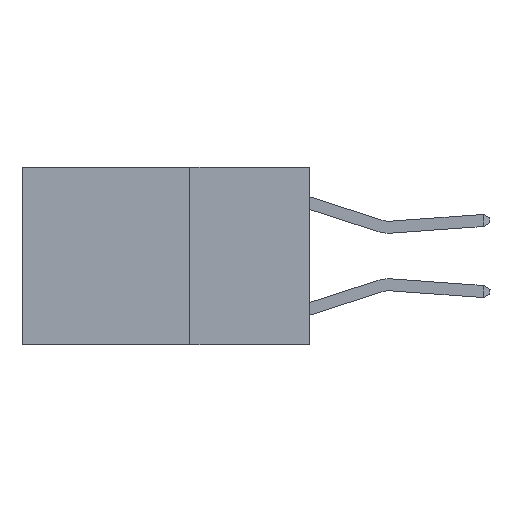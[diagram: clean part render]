
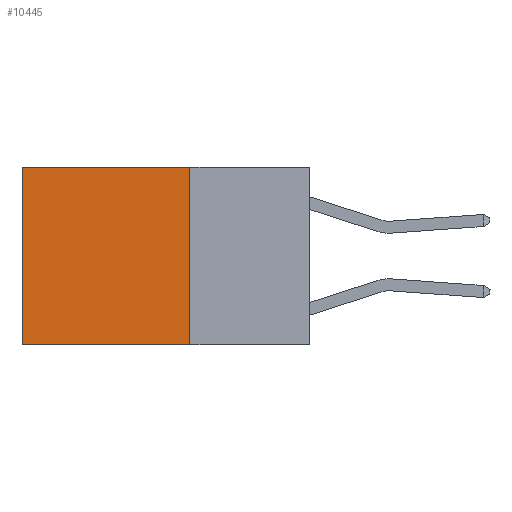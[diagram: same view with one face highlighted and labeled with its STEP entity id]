
A CAD part, left-side view. The second image highlights one B-rep face of the part: STEP entity #10445.
In plain terms, the highlighted planar face has unit normal (-1, 0, 0).
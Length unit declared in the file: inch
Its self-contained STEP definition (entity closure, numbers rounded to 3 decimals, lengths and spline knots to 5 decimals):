
#79 = CARTESIAN_POINT ( 'NONE',  ( 0.2625, 0.6, 0. ) ) ;
#118 = EDGE_LOOP ( 'NONE', ( #6776, #10476, #7624, #11613 ) ) ;
#320 = DIRECTION ( 'NONE',  ( 0., 1., 0. ) ) ;
#691 = EDGE_CURVE ( 'NONE', #8754, #4302, #3623, .T. ) ;
#780 = CARTESIAN_POINT ( 'NONE',  ( 0.2625, 0.25, 0. ) ) ;
#1047 = VECTOR ( 'NONE', #4508, 39.37008 ) ;
#1253 = CARTESIAN_POINT ( 'NONE',  ( 0.2625, 0.25, -0.37 ) ) ;
#2013 = DIRECTION ( 'NONE',  ( 0., 1., 0. ) ) ;
#2427 = VECTOR ( 'NONE', #2013, 39.37008 ) ;
#2598 = CARTESIAN_POINT ( 'NONE',  ( 0.2625, 0.25, 0. ) ) ;
#3438 = CARTESIAN_POINT ( 'NONE',  ( 0.2625, 0.6, 0. ) ) ;
#3510 = VERTEX_POINT ( 'NONE', #11440 ) ;
#3623 = LINE ( 'NONE', #79, #10559 ) ;
#3875 = LINE ( 'NONE', #1253, #6036 ) ;
#4302 = VERTEX_POINT ( 'NONE', #6297 ) ;
#4312 = EDGE_CURVE ( 'NONE', #4738, #3510, #8435, .T. ) ;
#4508 = DIRECTION ( 'NONE',  ( 0., 0., -1. ) ) ;
#4575 = DIRECTION ( 'NONE',  ( 0., 0., -1. ) ) ;
#4738 = VERTEX_POINT ( 'NONE', #11332 ) ;
#6036 = VECTOR ( 'NONE', #320, 39.37008 ) ;
#6297 = CARTESIAN_POINT ( 'NONE',  ( 0.2625, 0.6, -0.37 ) ) ;
#6776 = ORIENTED_EDGE ( 'NONE', *, *, #691, .T. ) ;
#6835 = FACE_OUTER_BOUND ( 'NONE', #118, .T. ) ;
#7290 = PLANE ( 'NONE',  #11433 ) ;
#7624 = ORIENTED_EDGE ( 'NONE', *, *, #4312, .F. ) ;
#8416 = EDGE_CURVE ( 'NONE', #4738, #8754, #9729, .T. ) ;
#8435 = LINE ( 'NONE', #2598, #1047 ) ;
#8754 = VERTEX_POINT ( 'NONE', #3438 ) ;
#9621 = EDGE_CURVE ( 'NONE', #3510, #4302, #3875, .T. ) ;
#9729 = LINE ( 'NONE', #11050, #2427 ) ;
#9971 = DIRECTION ( 'NONE',  ( 1., 0., 0. ) ) ;
#10178 = DIRECTION ( 'NONE',  ( 0., 0., -1. ) ) ;
#10445 = ADVANCED_FACE ( 'NONE', ( #6835 ), #7290, .F. ) ;
#10476 = ORIENTED_EDGE ( 'NONE', *, *, #9621, .F. ) ;
#10559 = VECTOR ( 'NONE', #10178, 39.37008 ) ;
#11050 = CARTESIAN_POINT ( 'NONE',  ( 0.2625, 0.25, 0. ) ) ;
#11332 = CARTESIAN_POINT ( 'NONE',  ( 0.2625, 0.25, 0. ) ) ;
#11433 = AXIS2_PLACEMENT_3D ( 'NONE', #780, #9971, #4575 ) ;
#11440 = CARTESIAN_POINT ( 'NONE',  ( 0.2625, 0.25, -0.37 ) ) ;
#11613 = ORIENTED_EDGE ( 'NONE', *, *, #8416, .T. ) ;
